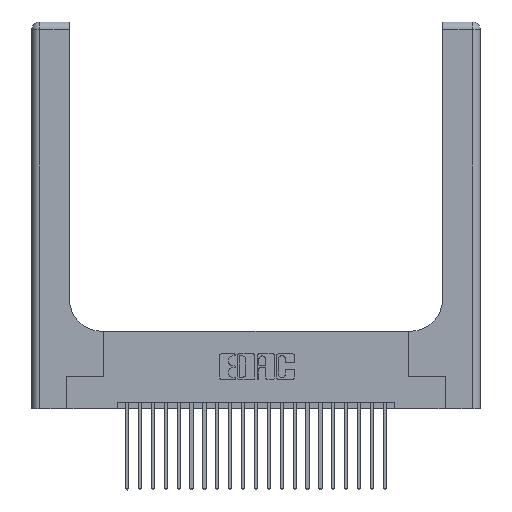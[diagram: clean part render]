
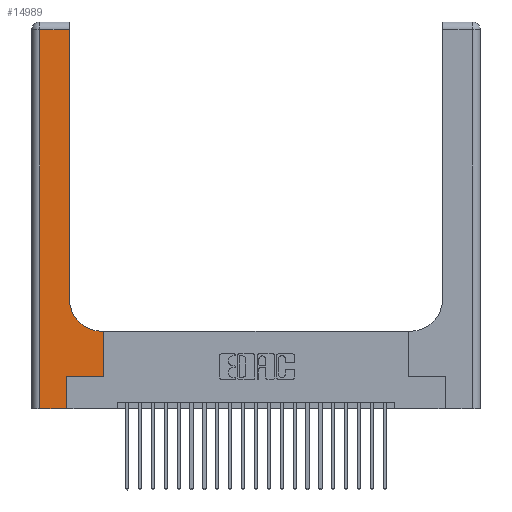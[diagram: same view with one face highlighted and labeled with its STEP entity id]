
A CAD part, top view. The second image highlights one B-rep face of the part: STEP entity #14989.
In plain terms, the highlighted planar face has unit normal (0, 0, 1).
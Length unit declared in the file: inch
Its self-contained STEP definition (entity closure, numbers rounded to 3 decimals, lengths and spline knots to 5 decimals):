
#76 = PLANE ( 'NONE',  #10287 ) ;
#1263 = CARTESIAN_POINT ( 'NONE',  ( 0., 0., 0.37 ) ) ;
#1509 = DIRECTION ( 'NONE',  ( -1., 0., 0. ) ) ;
#1610 = CARTESIAN_POINT ( 'NONE',  ( 0.06, 3., 0.37 ) ) ;
#1794 = ORIENTED_EDGE ( 'NONE', *, *, #6616, .T. ) ;
#2088 = EDGE_CURVE ( 'NONE', #8119, #2978, #18612, .T. ) ;
#2132 = VERTEX_POINT ( 'NONE', #16997 ) ;
#2978 = VERTEX_POINT ( 'NONE', #24505 ) ;
#3151 = CARTESIAN_POINT ( 'NONE',  ( 0.2915, 2.94, 0.37 ) ) ;
#4024 = EDGE_CURVE ( 'NONE', #24255, #11436, #4323, .T. ) ;
#4323 = LINE ( 'NONE', #1610, #23885 ) ;
#4900 = EDGE_CURVE ( 'NONE', #22350, #24255, #16099, .T. ) ;
#4975 = EDGE_CURVE ( 'NONE', #11305, #8119, #7781, .T. ) ;
#4991 = ORIENTED_EDGE ( 'NONE', *, *, #14166, .T. ) ;
#5158 = VECTOR ( 'NONE', #1509, 39.37008 ) ;
#5166 = CIRCLE ( 'NONE', #16288, 0.25 ) ;
#5488 = CARTESIAN_POINT ( 'NONE',  ( 0., 3., 0.37 ) ) ;
#5635 = ORIENTED_EDGE ( 'NONE', *, *, #16106, .T. ) ;
#5673 = CARTESIAN_POINT ( 'NONE',  ( 0.2915, 3., 0.37 ) ) ;
#5955 = LINE ( 'NONE', #17393, #23454 ) ;
#6147 = ORIENTED_EDGE ( 'NONE', *, *, #2088, .T. ) ;
#6232 = DIRECTION ( 'NONE',  ( 0., 1., 0. ) ) ;
#6455 = ORIENTED_EDGE ( 'NONE', *, *, #4024, .T. ) ;
#6616 = EDGE_CURVE ( 'NONE', #2978, #19434, #5955, .T. ) ;
#7028 = DIRECTION ( 'NONE',  ( 1., 0., 0. ) ) ;
#7157 = ORIENTED_EDGE ( 'NONE', *, *, #4900, .T. ) ;
#7781 = LINE ( 'NONE', #15076, #15486 ) ;
#8018 = CARTESIAN_POINT ( 'NONE',  ( 0.269, 0.25, 0.37 ) ) ;
#8045 = VECTOR ( 'NONE', #18918, 39.37008 ) ;
#8093 = FACE_OUTER_BOUND ( 'NONE', #18413, .T. ) ;
#8119 = VERTEX_POINT ( 'NONE', #19624 ) ;
#8432 = ORIENTED_EDGE ( 'NONE', *, *, #4975, .T. ) ;
#8751 = VECTOR ( 'NONE', #21445, 39.37008 ) ;
#10287 = AXIS2_PLACEMENT_3D ( 'NONE', #5488, #18791, #15103 ) ;
#10713 = CARTESIAN_POINT ( 'NONE',  ( 0.5415, 0.85, 0.37 ) ) ;
#10951 = DIRECTION ( 'NONE',  ( 0., 0., -1. ) ) ;
#11305 = VERTEX_POINT ( 'NONE', #16890 ) ;
#11436 = VERTEX_POINT ( 'NONE', #21686 ) ;
#11758 = EDGE_CURVE ( 'NONE', #21642, #2132, #5166, .T. ) ;
#12146 = CARTESIAN_POINT ( 'NONE',  ( 0.5415, 0.6, 0.37 ) ) ;
#12251 = CARTESIAN_POINT ( 'NONE',  ( 0.5585, 0.6, 0.37 ) ) ;
#12417 = VECTOR ( 'NONE', #7028, 39.37008 ) ;
#12684 = CARTESIAN_POINT ( 'NONE',  ( 0., 2.94, 0.37 ) ) ;
#12891 = CARTESIAN_POINT ( 'NONE',  ( 0.06, 2.94, 0.37 ) ) ;
#14166 = EDGE_CURVE ( 'NONE', #19434, #21642, #19087, .T. ) ;
#14509 = DIRECTION ( 'NONE',  ( 1., 0., 0. ) ) ;
#14599 = LINE ( 'NONE', #5673, #8045 ) ;
#14989 = ADVANCED_FACE ( 'NONE', ( #8093 ), #76, .F. ) ;
#15076 = CARTESIAN_POINT ( 'NONE',  ( 0.269, 0., 0.37 ) ) ;
#15103 = DIRECTION ( 'NONE',  ( -1., 0., 0. ) ) ;
#15486 = VECTOR ( 'NONE', #19062, 39.37008 ) ;
#15979 = VECTOR ( 'NONE', #14509, 39.37008 ) ;
#16099 = LINE ( 'NONE', #12684, #5158 ) ;
#16106 = EDGE_CURVE ( 'NONE', #2132, #22350, #14599, .T. ) ;
#16288 = AXIS2_PLACEMENT_3D ( 'NONE', #10713, #10951, #20346 ) ;
#16475 = ORIENTED_EDGE ( 'NONE', *, *, #18101, .T. ) ;
#16890 = CARTESIAN_POINT ( 'NONE',  ( 0.269, 0., 0.37 ) ) ;
#16997 = CARTESIAN_POINT ( 'NONE',  ( 0.2915, 0.85, 0.37 ) ) ;
#17393 = CARTESIAN_POINT ( 'NONE',  ( 0.5585, 0.25, 0.37 ) ) ;
#17777 = LINE ( 'NONE', #1263, #15979 ) ;
#18101 = EDGE_CURVE ( 'NONE', #11436, #11305, #17777, .T. ) ;
#18149 = DIRECTION ( 'NONE',  ( 0., -1., 0. ) ) ;
#18413 = EDGE_LOOP ( 'NONE', ( #5635, #7157, #6455, #16475, #8432, #6147, #1794, #4991, #19298 ) ) ;
#18612 = LINE ( 'NONE', #8018, #12417 ) ;
#18791 = DIRECTION ( 'NONE',  ( 0., 0., -1. ) ) ;
#18918 = DIRECTION ( 'NONE',  ( 0., 1., 0. ) ) ;
#19062 = DIRECTION ( 'NONE',  ( 0., 1., 0. ) ) ;
#19087 = LINE ( 'NONE', #19329, #8751 ) ;
#19298 = ORIENTED_EDGE ( 'NONE', *, *, #11758, .T. ) ;
#19329 = CARTESIAN_POINT ( 'NONE',  ( 0.2915, 0.6, 0.37 ) ) ;
#19434 = VERTEX_POINT ( 'NONE', #12251 ) ;
#19624 = CARTESIAN_POINT ( 'NONE',  ( 0.269, 0.25, 0.37 ) ) ;
#20346 = DIRECTION ( 'NONE',  ( 1., 0., 0. ) ) ;
#21445 = DIRECTION ( 'NONE',  ( -1., 0., 0. ) ) ;
#21642 = VERTEX_POINT ( 'NONE', #12146 ) ;
#21686 = CARTESIAN_POINT ( 'NONE',  ( 0.06, 0., 0.37 ) ) ;
#22350 = VERTEX_POINT ( 'NONE', #3151 ) ;
#23454 = VECTOR ( 'NONE', #6232, 39.37008 ) ;
#23885 = VECTOR ( 'NONE', #18149, 39.37008 ) ;
#24255 = VERTEX_POINT ( 'NONE', #12891 ) ;
#24505 = CARTESIAN_POINT ( 'NONE',  ( 0.5585, 0.25, 0.37 ) ) ;
